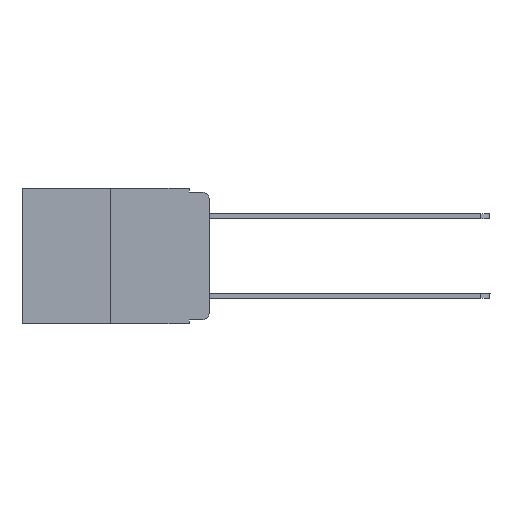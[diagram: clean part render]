
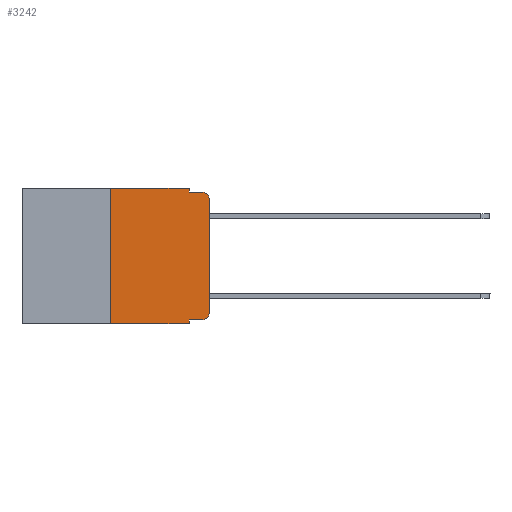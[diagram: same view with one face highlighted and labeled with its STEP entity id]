
A CAD part, left-side view. The second image highlights one B-rep face of the part: STEP entity #3242.
In plain terms, the highlighted planar face has unit normal (-1, 0, 0).
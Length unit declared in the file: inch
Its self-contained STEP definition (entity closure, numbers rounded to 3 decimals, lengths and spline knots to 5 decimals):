
#50 = LINE ( 'NONE', #4271, #12844 ) ;
#110 = VECTOR ( 'NONE', #1684, 39.37008 ) ;
#162 = AXIS2_PLACEMENT_3D ( 'NONE', #12215, #8112, #11382 ) ;
#271 = EDGE_CURVE ( 'NONE', #5947, #5441, #7262, .T. ) ;
#407 = CARTESIAN_POINT ( 'NONE',  ( 0., 0.02, -0.01 ) ) ;
#1230 = VECTOR ( 'NONE', #6367, 39.37008 ) ;
#1382 = CARTESIAN_POINT ( 'NONE',  ( 0., 0., 0. ) ) ;
#1460 = VECTOR ( 'NONE', #2639, 39.37008 ) ;
#1594 = DIRECTION ( 'NONE',  ( 0., 0., -1. ) ) ;
#1630 = LINE ( 'NONE', #9036, #13357 ) ;
#1684 = DIRECTION ( 'NONE',  ( 0., -1., 0. ) ) ;
#1805 = PLANE ( 'NONE',  #10660 ) ;
#2172 = LINE ( 'NONE', #8337, #1230 ) ;
#2438 = VERTEX_POINT ( 'NONE', #11868 ) ;
#2639 = DIRECTION ( 'NONE',  ( 0., -1., 0. ) ) ;
#2767 = VERTEX_POINT ( 'NONE', #3142 ) ;
#2782 = VECTOR ( 'NONE', #8593, 39.37008 ) ;
#3116 = EDGE_CURVE ( 'NONE', #2767, #5660, #50, .T. ) ;
#3128 = EDGE_CURVE ( 'NONE', #3437, #2438, #10774, .T. ) ;
#3132 = VERTEX_POINT ( 'NONE', #407 ) ;
#3142 = CARTESIAN_POINT ( 'NONE',  ( 0., 0.051, -0.333 ) ) ;
#3242 = ADVANCED_FACE ( 'NONE', ( #7919 ), #1805, .F. ) ;
#3437 = VERTEX_POINT ( 'NONE', #5522 ) ;
#3455 = CARTESIAN_POINT ( 'NONE',  ( 0., 0.473, 0. ) ) ;
#3587 = DIRECTION ( 'NONE',  ( 1., 0., 0. ) ) ;
#3639 = DIRECTION ( 'NONE',  ( -1., 0., 0. ) ) ;
#3691 = DIRECTION ( 'NONE',  ( 0., -1., 0. ) ) ;
#4271 = CARTESIAN_POINT ( 'NONE',  ( 0., 0.051, -0.333 ) ) ;
#4387 = CIRCLE ( 'NONE', #12055, 0.02 ) ;
#4582 = EDGE_CURVE ( 'NONE', #5660, #3437, #4387, .T. ) ;
#4824 = ORIENTED_EDGE ( 'NONE', *, *, #10479, .T. ) ;
#4857 = EDGE_CURVE ( 'NONE', #5441, #9858, #7724, .T. ) ;
#4917 = CARTESIAN_POINT ( 'NONE',  ( 0., 0.473, -0.343 ) ) ;
#5428 = ORIENTED_EDGE ( 'NONE', *, *, #4582, .T. ) ;
#5441 = VERTEX_POINT ( 'NONE', #13251 ) ;
#5522 = CARTESIAN_POINT ( 'NONE',  ( 0., 0., -0.313 ) ) ;
#5660 = VERTEX_POINT ( 'NONE', #13155 ) ;
#5811 = LINE ( 'NONE', #4917, #110 ) ;
#5947 = VERTEX_POINT ( 'NONE', #6418 ) ;
#6266 = EDGE_LOOP ( 'NONE', ( #8397, #11559, #12785, #12804, #13218, #11541, #4824, #7030, #8752, #5428 ) ) ;
#6367 = DIRECTION ( 'NONE',  ( 0., 0., -1. ) ) ;
#6418 = CARTESIAN_POINT ( 'NONE',  ( 0., 0.25, -0.343 ) ) ;
#6650 = EDGE_CURVE ( 'NONE', #2767, #12573, #7835, .T. ) ;
#6662 = DIRECTION ( 'NONE',  ( 0., 0., -1. ) ) ;
#6736 = EDGE_CURVE ( 'NONE', #2438, #3132, #9590, .T. ) ;
#7030 = ORIENTED_EDGE ( 'NONE', *, *, #6650, .F. ) ;
#7100 = DIRECTION ( 'NONE',  ( 0., -1., 0. ) ) ;
#7262 = LINE ( 'NONE', #11430, #10669 ) ;
#7724 = LINE ( 'NONE', #3455, #1460 ) ;
#7835 = LINE ( 'NONE', #12017, #9365 ) ;
#7919 = FACE_OUTER_BOUND ( 'NONE', #6266, .T. ) ;
#8112 = DIRECTION ( 'NONE',  ( -1., 0., 0. ) ) ;
#8337 = CARTESIAN_POINT ( 'NONE',  ( 0., 0.051, 0. ) ) ;
#8397 = ORIENTED_EDGE ( 'NONE', *, *, #3128, .T. ) ;
#8593 = DIRECTION ( 'NONE',  ( 0., 0., 1. ) ) ;
#8648 = CARTESIAN_POINT ( 'NONE',  ( 0., 0.051, -0.343 ) ) ;
#8752 = ORIENTED_EDGE ( 'NONE', *, *, #3116, .T. ) ;
#8849 = CARTESIAN_POINT ( 'NONE',  ( 0., 0.02, -0.313 ) ) ;
#8857 = CARTESIAN_POINT ( 'NONE',  ( 0., 0.473, 0. ) ) ;
#9036 = CARTESIAN_POINT ( 'NONE',  ( 0., 0.051, -0.01 ) ) ;
#9086 = CARTESIAN_POINT ( 'NONE',  ( 0., 0.051, -0.01 ) ) ;
#9238 = CARTESIAN_POINT ( 'NONE',  ( 0., 0.051, 0. ) ) ;
#9289 = DIRECTION ( 'NONE',  ( 0., 0., 1. ) ) ;
#9365 = VECTOR ( 'NONE', #1594, 39.37008 ) ;
#9590 = CIRCLE ( 'NONE', #162, 0.02 ) ;
#9858 = VERTEX_POINT ( 'NONE', #9238 ) ;
#10130 = VERTEX_POINT ( 'NONE', #9086 ) ;
#10253 = EDGE_CURVE ( 'NONE', #9858, #10130, #2172, .T. ) ;
#10479 = EDGE_CURVE ( 'NONE', #5947, #12573, #5811, .T. ) ;
#10660 = AXIS2_PLACEMENT_3D ( 'NONE', #8857, #3587, #13041 ) ;
#10669 = VECTOR ( 'NONE', #9289, 39.37008 ) ;
#10774 = LINE ( 'NONE', #1382, #2782 ) ;
#11382 = DIRECTION ( 'NONE',  ( 0., 0., -1. ) ) ;
#11430 = CARTESIAN_POINT ( 'NONE',  ( 0., 0.25, 0. ) ) ;
#11541 = ORIENTED_EDGE ( 'NONE', *, *, #271, .F. ) ;
#11559 = ORIENTED_EDGE ( 'NONE', *, *, #6736, .T. ) ;
#11868 = CARTESIAN_POINT ( 'NONE',  ( 0., 0., -0.03 ) ) ;
#12017 = CARTESIAN_POINT ( 'NONE',  ( 0., 0.051, 0. ) ) ;
#12055 = AXIS2_PLACEMENT_3D ( 'NONE', #8849, #3639, #6662 ) ;
#12215 = CARTESIAN_POINT ( 'NONE',  ( 0., 0.02, -0.03 ) ) ;
#12573 = VERTEX_POINT ( 'NONE', #8648 ) ;
#12785 = ORIENTED_EDGE ( 'NONE', *, *, #13037, .F. ) ;
#12804 = ORIENTED_EDGE ( 'NONE', *, *, #10253, .F. ) ;
#12844 = VECTOR ( 'NONE', #7100, 39.37008 ) ;
#13037 = EDGE_CURVE ( 'NONE', #10130, #3132, #1630, .T. ) ;
#13041 = DIRECTION ( 'NONE',  ( 0., 0., -1. ) ) ;
#13155 = CARTESIAN_POINT ( 'NONE',  ( 0., 0.02, -0.333 ) ) ;
#13218 = ORIENTED_EDGE ( 'NONE', *, *, #4857, .F. ) ;
#13251 = CARTESIAN_POINT ( 'NONE',  ( 0., 0.25, 0. ) ) ;
#13357 = VECTOR ( 'NONE', #3691, 39.37008 ) ;
